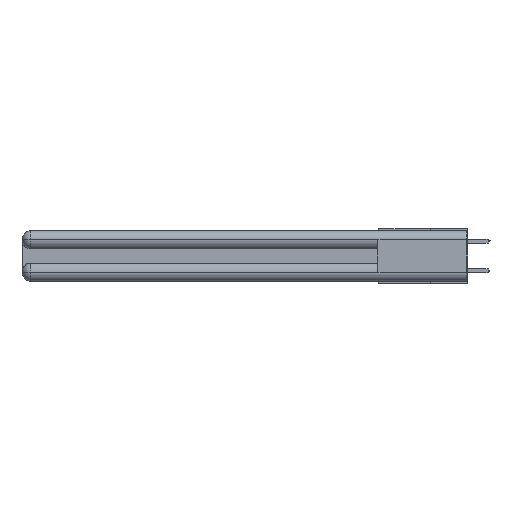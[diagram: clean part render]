
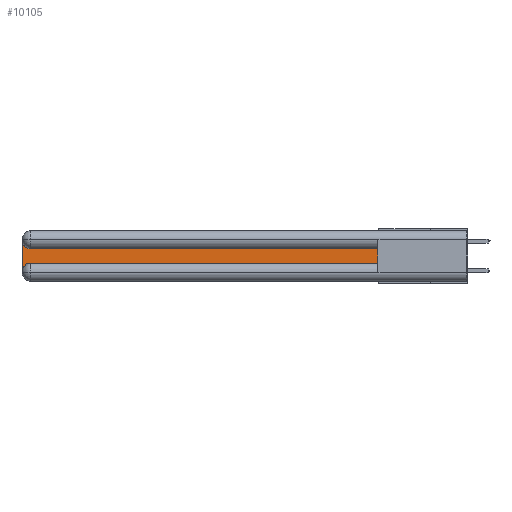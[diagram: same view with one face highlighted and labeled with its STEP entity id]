
A CAD part, left-side view. The second image highlights one B-rep face of the part: STEP entity #10105.
In plain terms, the highlighted planar face has unit normal (-1, 0, 0).
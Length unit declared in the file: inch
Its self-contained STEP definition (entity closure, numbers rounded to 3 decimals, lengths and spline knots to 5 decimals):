
#330 = CARTESIAN_POINT ( 'NONE',  ( 0.075, 2.94, -0.1225 ) ) ;
#546 = FACE_OUTER_BOUND ( 'NONE', #21172, .T. ) ;
#680 = DIRECTION ( 'NONE',  ( 1., 0., 0. ) ) ;
#840 = VECTOR ( 'NONE', #15823, 39.37008 ) ;
#1667 = ORIENTED_EDGE ( 'NONE', *, *, #11110, .T. ) ;
#1804 = VERTEX_POINT ( 'NONE', #18603 ) ;
#3649 = CIRCLE ( 'NONE', #18388, 0.06 ) ;
#4398 = EDGE_CURVE ( 'NONE', #25785, #29156, #14019, .T. ) ;
#4673 = DIRECTION ( 'NONE',  ( 0., 0., -1. ) ) ;
#4734 = CARTESIAN_POINT ( 'NONE',  ( 0.075, 3., -0.1225 ) ) ;
#5048 = EDGE_CURVE ( 'NONE', #23560, #24965, #8343, .T. ) ;
#5586 = ORIENTED_EDGE ( 'NONE', *, *, #26710, .T. ) ;
#8132 = CARTESIAN_POINT ( 'NONE',  ( 0.075, 0.6, -0.1225 ) ) ;
#8343 = LINE ( 'NONE', #17197, #26443 ) ;
#9609 = CARTESIAN_POINT ( 'NONE',  ( 0.075, 3., -0.2775 ) ) ;
#10101 = ORIENTED_EDGE ( 'NONE', *, *, #4398, .T. ) ;
#10105 = ADVANCED_FACE ( 'NONE', ( #546 ), #16129, .F. ) ;
#11110 = EDGE_CURVE ( 'NONE', #1804, #25785, #22508, .T. ) ;
#13585 = DIRECTION ( 'NONE',  ( 1., 0., 0. ) ) ;
#13744 = DIRECTION ( 'NONE',  ( 0., 0., -1. ) ) ;
#14019 = CIRCLE ( 'NONE', #15064, 0.06 ) ;
#14306 = EDGE_CURVE ( 'NONE', #29156, #24981, #21307, .T. ) ;
#14308 = ORIENTED_EDGE ( 'NONE', *, *, #5048, .T. ) ;
#14933 = ORIENTED_EDGE ( 'NONE', *, *, #28686, .T. ) ;
#15064 = AXIS2_PLACEMENT_3D ( 'NONE', #28091, #680, #16589 ) ;
#15823 = DIRECTION ( 'NONE',  ( 0., 0., -1. ) ) ;
#16129 = PLANE ( 'NONE',  #20773 ) ;
#16589 = DIRECTION ( 'NONE',  ( 0., 0., -1. ) ) ;
#17197 = CARTESIAN_POINT ( 'NONE',  ( 0.075, 0.6, -0.1225 ) ) ;
#18032 = DIRECTION ( 'NONE',  ( 1., 0., 0. ) ) ;
#18388 = AXIS2_PLACEMENT_3D ( 'NONE', #25100, #13585, #4673 ) ;
#18603 = CARTESIAN_POINT ( 'NONE',  ( 0.075, 3., -0.0625 ) ) ;
#19155 = VECTOR ( 'NONE', #21593, 39.37008 ) ;
#19229 = CARTESIAN_POINT ( 'NONE',  ( 0.075, 0.6, -0.2175 ) ) ;
#20013 = CARTESIAN_POINT ( 'NONE',  ( 0.075, 3., -0.2175 ) ) ;
#20616 = VECTOR ( 'NONE', #26131, 39.37008 ) ;
#20773 = AXIS2_PLACEMENT_3D ( 'NONE', #4734, #18032, #13744 ) ;
#21172 = EDGE_LOOP ( 'NONE', ( #14308, #5586, #1667, #10101, #23341, #14933 ) ) ;
#21307 = LINE ( 'NONE', #25931, #20616 ) ;
#21441 = DIRECTION ( 'NONE',  ( 0., 1., 0. ) ) ;
#21593 = DIRECTION ( 'NONE',  ( 0., 0., 1. ) ) ;
#22508 = LINE ( 'NONE', #20013, #840 ) ;
#23188 = CARTESIAN_POINT ( 'NONE',  ( 0.075, 0.6, -0.2175 ) ) ;
#23341 = ORIENTED_EDGE ( 'NONE', *, *, #14306, .T. ) ;
#23560 = VERTEX_POINT ( 'NONE', #8132 ) ;
#24965 = VERTEX_POINT ( 'NONE', #330 ) ;
#24981 = VERTEX_POINT ( 'NONE', #23188 ) ;
#25100 = CARTESIAN_POINT ( 'NONE',  ( 0.075, 2.94, -0.0625 ) ) ;
#25785 = VERTEX_POINT ( 'NONE', #9609 ) ;
#25884 = LINE ( 'NONE', #19229, #19155 ) ;
#25931 = CARTESIAN_POINT ( 'NONE',  ( 0.075, 0.6, -0.2175 ) ) ;
#26131 = DIRECTION ( 'NONE',  ( 0., -1., 0. ) ) ;
#26443 = VECTOR ( 'NONE', #21441, 39.37008 ) ;
#26710 = EDGE_CURVE ( 'NONE', #24965, #1804, #3649, .T. ) ;
#28091 = CARTESIAN_POINT ( 'NONE',  ( 0.075, 2.94, -0.2775 ) ) ;
#28654 = CARTESIAN_POINT ( 'NONE',  ( 0.075, 2.94, -0.2175 ) ) ;
#28686 = EDGE_CURVE ( 'NONE', #24981, #23560, #25884, .T. ) ;
#29156 = VERTEX_POINT ( 'NONE', #28654 ) ;
